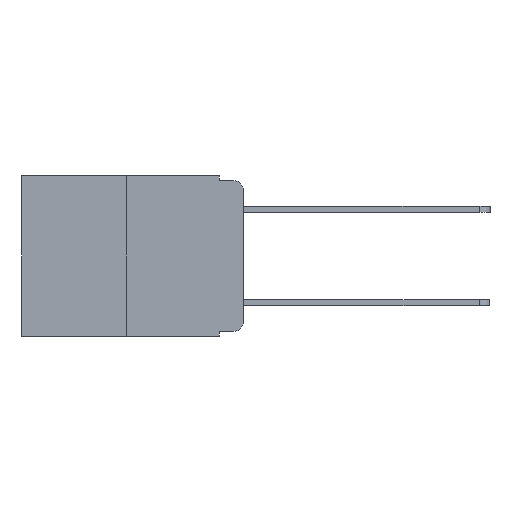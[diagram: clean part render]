
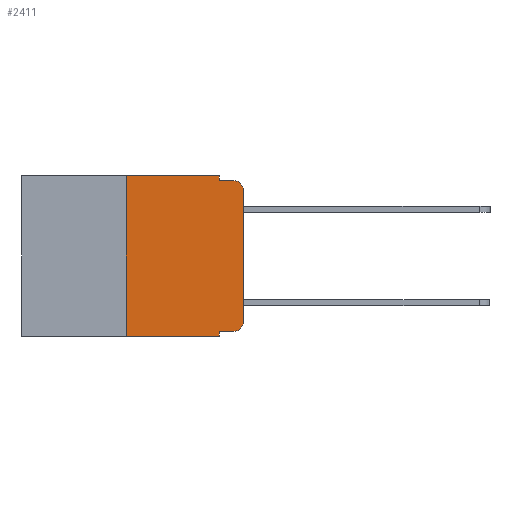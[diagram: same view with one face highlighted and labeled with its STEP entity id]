
A CAD part, left-side view. The second image highlights one B-rep face of the part: STEP entity #2411.
In plain terms, the highlighted planar face has unit normal (-1, 0, 0).
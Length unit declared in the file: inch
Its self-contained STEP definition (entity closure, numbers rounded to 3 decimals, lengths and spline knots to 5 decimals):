
#166 = DIRECTION ( 'NONE',  ( 0., -1., 0. ) ) ;
#231 = CARTESIAN_POINT ( 'NONE',  ( 0., 0.051, -0.343 ) ) ;
#706 = EDGE_CURVE ( 'NONE', #12650, #10285, #4537, .T. ) ;
#869 = VERTEX_POINT ( 'NONE', #6482 ) ;
#1104 = ORIENTED_EDGE ( 'NONE', *, *, #2689, .F. ) ;
#1334 = ORIENTED_EDGE ( 'NONE', *, *, #13520, .F. ) ;
#1545 = VECTOR ( 'NONE', #2578, 39.37008 ) ;
#1602 = ORIENTED_EDGE ( 'NONE', *, *, #12863, .F. ) ;
#2260 = EDGE_CURVE ( 'NONE', #8140, #10285, #9863, .T. ) ;
#2411 = ADVANCED_FACE ( 'NONE', ( #10591 ), #7223, .F. ) ;
#2462 = CARTESIAN_POINT ( 'NONE',  ( 0., 0.25, 0. ) ) ;
#2578 = DIRECTION ( 'NONE',  ( 0., -1., 0. ) ) ;
#2689 = EDGE_CURVE ( 'NONE', #4440, #12012, #4983, .T. ) ;
#2760 = VECTOR ( 'NONE', #166, 39.37008 ) ;
#3027 = EDGE_CURVE ( 'NONE', #8056, #8140, #12608, .T. ) ;
#3352 = AXIS2_PLACEMENT_3D ( 'NONE', #7885, #7986, #8042 ) ;
#4077 = VERTEX_POINT ( 'NONE', #11461 ) ;
#4283 = CARTESIAN_POINT ( 'NONE',  ( 0., 0.051, -0.01 ) ) ;
#4440 = VERTEX_POINT ( 'NONE', #7948 ) ;
#4513 = CARTESIAN_POINT ( 'NONE',  ( 0., 0., 0. ) ) ;
#4537 = LINE ( 'NONE', #12777, #1545 ) ;
#4788 = DIRECTION ( 'NONE',  ( -1., 0., 0. ) ) ;
#4814 = VECTOR ( 'NONE', #7974, 39.37008 ) ;
#4906 = ORIENTED_EDGE ( 'NONE', *, *, #2260, .T. ) ;
#4983 = LINE ( 'NONE', #12316, #12667 ) ;
#5069 = CARTESIAN_POINT ( 'NONE',  ( 0., 0.051, 0. ) ) ;
#5117 = ORIENTED_EDGE ( 'NONE', *, *, #11583, .F. ) ;
#5178 = CARTESIAN_POINT ( 'NONE',  ( 0., 0.473, 0. ) ) ;
#5211 = ORIENTED_EDGE ( 'NONE', *, *, #10937, .T. ) ;
#5321 = CARTESIAN_POINT ( 'NONE',  ( 0., 0.051, 0. ) ) ;
#5327 = LINE ( 'NONE', #2462, #8460 ) ;
#5700 = VECTOR ( 'NONE', #7748, 39.37008 ) ;
#5713 = ORIENTED_EDGE ( 'NONE', *, *, #706, .F. ) ;
#5953 = EDGE_CURVE ( 'NONE', #10960, #5979, #11039, .T. ) ;
#5979 = VERTEX_POINT ( 'NONE', #231 ) ;
#6482 = CARTESIAN_POINT ( 'NONE',  ( 0., 0.02, -0.333 ) ) ;
#6699 = CARTESIAN_POINT ( 'NONE',  ( 0., 0.051, -0.333 ) ) ;
#7223 = PLANE ( 'NONE',  #11621 ) ;
#7666 = DIRECTION ( 'NONE',  ( 0., 0., -1. ) ) ;
#7707 = DIRECTION ( 'NONE',  ( 1., 0., 0. ) ) ;
#7748 = DIRECTION ( 'NONE',  ( 0., -1., 0. ) ) ;
#7885 = CARTESIAN_POINT ( 'NONE',  ( 0., 0.02, -0.03 ) ) ;
#7919 = CARTESIAN_POINT ( 'NONE',  ( 0., 0.473, -0.343 ) ) ;
#7948 = CARTESIAN_POINT ( 'NONE',  ( 0., 0.25, 0. ) ) ;
#7974 = DIRECTION ( 'NONE',  ( 0., 0., -1. ) ) ;
#7986 = DIRECTION ( 'NONE',  ( -1., 0., 0. ) ) ;
#8042 = DIRECTION ( 'NONE',  ( 0., 0., -1. ) ) ;
#8056 = VERTEX_POINT ( 'NONE', #8818 ) ;
#8140 = VERTEX_POINT ( 'NONE', #10983 ) ;
#8460 = VECTOR ( 'NONE', #9883, 39.37008 ) ;
#8818 = CARTESIAN_POINT ( 'NONE',  ( 0., 0., -0.313 ) ) ;
#9688 = DIRECTION ( 'NONE',  ( 0., 0., 1. ) ) ;
#9863 = CIRCLE ( 'NONE', #3352, 0.02 ) ;
#9883 = DIRECTION ( 'NONE',  ( 0., 0., 1. ) ) ;
#10032 = LINE ( 'NONE', #5321, #12241 ) ;
#10102 = VECTOR ( 'NONE', #9688, 39.37008 ) ;
#10285 = VERTEX_POINT ( 'NONE', #10804 ) ;
#10327 = EDGE_CURVE ( 'NONE', #869, #8056, #11835, .T. ) ;
#10557 = ORIENTED_EDGE ( 'NONE', *, *, #10327, .T. ) ;
#10591 = FACE_OUTER_BOUND ( 'NONE', #11155, .T. ) ;
#10752 = CARTESIAN_POINT ( 'NONE',  ( 0., 0.25, -0.343 ) ) ;
#10804 = CARTESIAN_POINT ( 'NONE',  ( 0., 0.02, -0.01 ) ) ;
#10883 = CARTESIAN_POINT ( 'NONE',  ( 0., 0.02, -0.313 ) ) ;
#10927 = CARTESIAN_POINT ( 'NONE',  ( 0., 0.051, 0. ) ) ;
#10937 = EDGE_CURVE ( 'NONE', #4077, #869, #11058, .T. ) ;
#10960 = VERTEX_POINT ( 'NONE', #10752 ) ;
#10983 = CARTESIAN_POINT ( 'NONE',  ( 0., 0., -0.03 ) ) ;
#11039 = LINE ( 'NONE', #7919, #2760 ) ;
#11058 = LINE ( 'NONE', #6699, #5700 ) ;
#11155 = EDGE_LOOP ( 'NONE', ( #12216, #4906, #5713, #1334, #1104, #1602, #12754, #5117, #5211, #10557 ) ) ;
#11461 = CARTESIAN_POINT ( 'NONE',  ( 0., 0.051, -0.333 ) ) ;
#11583 = EDGE_CURVE ( 'NONE', #4077, #5979, #10032, .T. ) ;
#11621 = AXIS2_PLACEMENT_3D ( 'NONE', #5178, #7707, #7666 ) ;
#11835 = CIRCLE ( 'NONE', #11849, 0.02 ) ;
#11844 = DIRECTION ( 'NONE',  ( 0., 0., -1. ) ) ;
#11849 = AXIS2_PLACEMENT_3D ( 'NONE', #10883, #4788, #11844 ) ;
#12012 = VERTEX_POINT ( 'NONE', #5069 ) ;
#12063 = DIRECTION ( 'NONE',  ( 0., -1., 0. ) ) ;
#12216 = ORIENTED_EDGE ( 'NONE', *, *, #3027, .T. ) ;
#12241 = VECTOR ( 'NONE', #12330, 39.37008 ) ;
#12316 = CARTESIAN_POINT ( 'NONE',  ( 0., 0.473, 0. ) ) ;
#12330 = DIRECTION ( 'NONE',  ( 0., 0., -1. ) ) ;
#12608 = LINE ( 'NONE', #4513, #10102 ) ;
#12650 = VERTEX_POINT ( 'NONE', #4283 ) ;
#12667 = VECTOR ( 'NONE', #12063, 39.37008 ) ;
#12754 = ORIENTED_EDGE ( 'NONE', *, *, #5953, .T. ) ;
#12777 = CARTESIAN_POINT ( 'NONE',  ( 0., 0.051, -0.01 ) ) ;
#12806 = LINE ( 'NONE', #10927, #4814 ) ;
#12863 = EDGE_CURVE ( 'NONE', #10960, #4440, #5327, .T. ) ;
#13520 = EDGE_CURVE ( 'NONE', #12012, #12650, #12806, .T. ) ;
